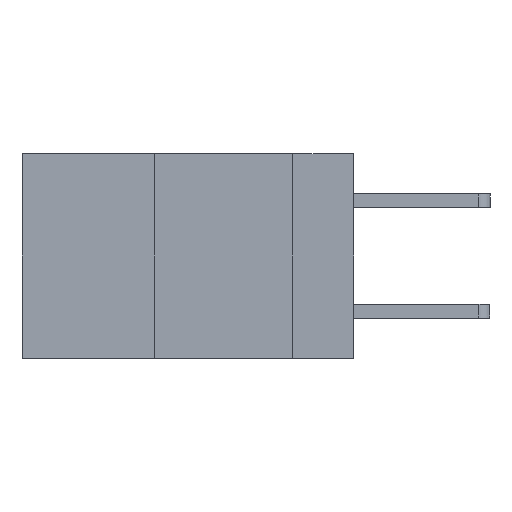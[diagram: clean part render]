
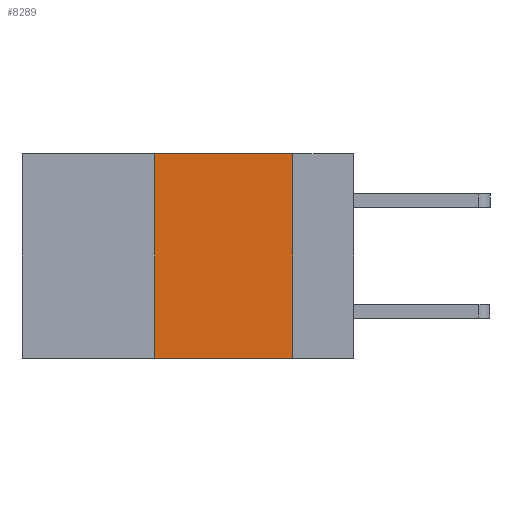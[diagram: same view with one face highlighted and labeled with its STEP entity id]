
A CAD part, left-side view. The second image highlights one B-rep face of the part: STEP entity #8289.
In plain terms, the highlighted planar face has unit normal (-1, 0, 0).
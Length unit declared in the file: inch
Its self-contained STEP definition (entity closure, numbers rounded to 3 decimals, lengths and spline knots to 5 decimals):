
#106 = CARTESIAN_POINT ( 'NONE',  ( 0., 0.11, -0.37 ) ) ;
#516 = LINE ( 'NONE', #2263, #6912 ) ;
#768 = CARTESIAN_POINT ( 'NONE',  ( 0., 0.6, 0. ) ) ;
#829 = DIRECTION ( 'NONE',  ( 0., 0., -1. ) ) ;
#1104 = EDGE_CURVE ( 'NONE', #9105, #7055, #4579, .T. ) ;
#1503 = DIRECTION ( 'NONE',  ( 0., -1., 0. ) ) ;
#1833 = CARTESIAN_POINT ( 'NONE',  ( 0., 0.11, 0. ) ) ;
#2263 = CARTESIAN_POINT ( 'NONE',  ( 0., 0.11, 0. ) ) ;
#2671 = ORIENTED_EDGE ( 'NONE', *, *, #8649, .F. ) ;
#3046 = CARTESIAN_POINT ( 'NONE',  ( 0., 0.36, 0. ) ) ;
#3503 = ORIENTED_EDGE ( 'NONE', *, *, #1104, .F. ) ;
#3770 = PLANE ( 'NONE',  #7747 ) ;
#3873 = DIRECTION ( 'NONE',  ( 0., 0., 1. ) ) ;
#4166 = EDGE_CURVE ( 'NONE', #4616, #8502, #8928, .T. ) ;
#4339 = CARTESIAN_POINT ( 'NONE',  ( 0., 0.6, 0. ) ) ;
#4579 = LINE ( 'NONE', #768, #4868 ) ;
#4616 = VERTEX_POINT ( 'NONE', #8961 ) ;
#4868 = VECTOR ( 'NONE', #1503, 39.37008 ) ;
#5028 = DIRECTION ( 'NONE',  ( 0., -1., 0. ) ) ;
#5134 = CARTESIAN_POINT ( 'NONE',  ( 0., 0.6, -0.37 ) ) ;
#5424 = EDGE_LOOP ( 'NONE', ( #2671, #3503, #8189, #5427 ) ) ;
#5427 = ORIENTED_EDGE ( 'NONE', *, *, #4166, .T. ) ;
#6364 = VECTOR ( 'NONE', #5028, 39.37008 ) ;
#6405 = LINE ( 'NONE', #7931, #9192 ) ;
#6747 = DIRECTION ( 'NONE',  ( 0., 0., -1. ) ) ;
#6812 = FACE_OUTER_BOUND ( 'NONE', #5424, .T. ) ;
#6912 = VECTOR ( 'NONE', #6747, 39.37008 ) ;
#7055 = VERTEX_POINT ( 'NONE', #1833 ) ;
#7502 = DIRECTION ( 'NONE',  ( 1., 0., 0. ) ) ;
#7747 = AXIS2_PLACEMENT_3D ( 'NONE', #4339, #7502, #829 ) ;
#7849 = EDGE_CURVE ( 'NONE', #4616, #9105, #6405, .T. ) ;
#7931 = CARTESIAN_POINT ( 'NONE',  ( 0., 0.36, 0. ) ) ;
#8189 = ORIENTED_EDGE ( 'NONE', *, *, #7849, .F. ) ;
#8289 = ADVANCED_FACE ( 'NONE', ( #6812 ), #3770, .F. ) ;
#8502 = VERTEX_POINT ( 'NONE', #106 ) ;
#8649 = EDGE_CURVE ( 'NONE', #7055, #8502, #516, .T. ) ;
#8928 = LINE ( 'NONE', #5134, #6364 ) ;
#8961 = CARTESIAN_POINT ( 'NONE',  ( 0., 0.36, -0.37 ) ) ;
#9105 = VERTEX_POINT ( 'NONE', #3046 ) ;
#9192 = VECTOR ( 'NONE', #3873, 39.37008 ) ;
